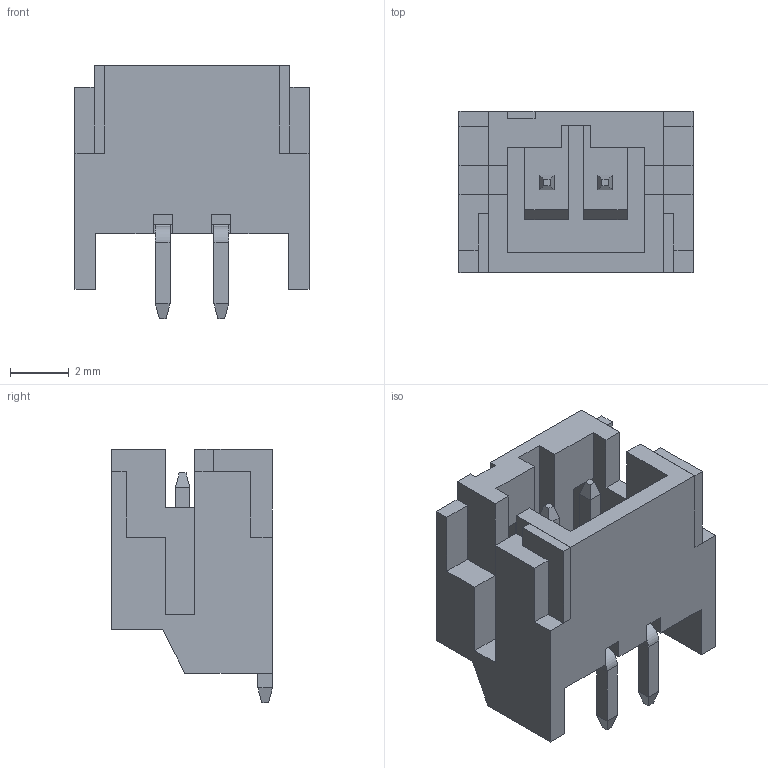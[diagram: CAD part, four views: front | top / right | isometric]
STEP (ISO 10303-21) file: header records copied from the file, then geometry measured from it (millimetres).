
FILE_DESCRIPTION (( 'STEP AP203' ), '1' );
FILE_NAME ('140-502-417-060.STEP', '2020-03-31T20:18:47', ( '' ), ( '' ), 'SwSTEP 2.0', 'SolidWorks 2016', '' );
FILE_SCHEMA (( 'CONFIG_CONTROL_DESIGN' ));
Length unit declared in the file: millimetre
Products named in the file (4): RA SMT Housing_502; RA SMT Pad; 140-502-417-060; RA SMT Contact
Assembly tree (5 placements, depth 2):
  140-502-417-060
    RA SMT Housing_502
    RA SMT Contact  x2
    RA SMT Pad  x2
Bounding box: 8 x 5.5 x 8.65 mm (x, y, z)
Volume: 142.3 mm3; surface area: 488.9 mm2
Topology: 5 solids, 5 shells, 172 faces, 448 edges, 282 vertices
Faces by surface type: plane 164, cylinder 8
Entity records: 4714 total; most frequent: CARTESIAN_POINT 762, ORIENTED_EDGE 752, DIRECTION 672, EDGE_CURVE 376, LINE 368, VECTOR 368, VERTEX_POINT 242, AXIS2_PLACEMENT_3D 152
